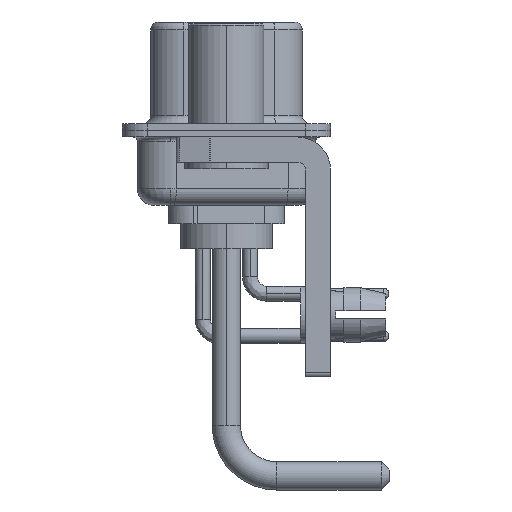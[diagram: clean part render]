
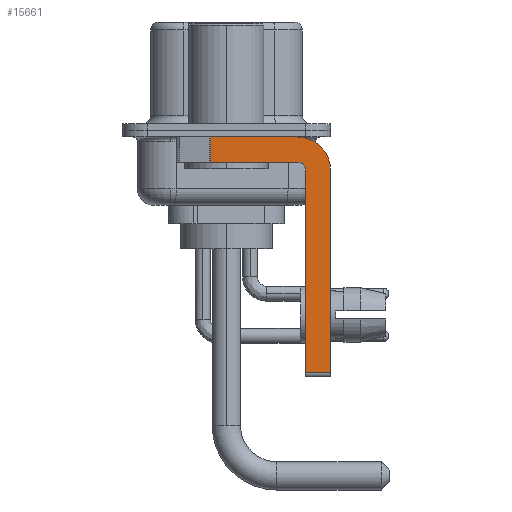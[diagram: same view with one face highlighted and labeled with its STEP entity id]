
A CAD part, left-side view. The second image highlights one B-rep face of the part: STEP entity #15661.
In plain terms, the highlighted planar face has unit normal (-1, 0, 0).
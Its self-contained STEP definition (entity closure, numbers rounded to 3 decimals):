
#631 = LINE ( 'NONE', #7253, #27463 ) ;
#889 = CARTESIAN_POINT ( 'NONE',  ( -2.9, -6.25, -2.4 ) ) ;
#1172 = CARTESIAN_POINT ( 'NONE',  ( -2.9, -4.25, -1.9 ) ) ;
#1406 = CARTESIAN_POINT ( 'NONE',  ( -2.9, 0.978, -0.4 ) ) ;
#1582 = CARTESIAN_POINT ( 'NONE',  ( -2.9, -6.25, -14.55 ) ) ;
#1620 = ORIENTED_EDGE ( 'NONE', *, *, #12519, .T. ) ;
#1623 = LINE ( 'NONE', #1172, #14168 ) ;
#1681 = CARTESIAN_POINT ( 'NONE',  ( -2.9, -4.25, -0.4 ) ) ;
#2259 = CARTESIAN_POINT ( 'NONE',  ( -2.9, -4.75, -14.55 ) ) ;
#2605 = FACE_OUTER_BOUND ( 'NONE', #25635, .T. ) ;
#3520 = AXIS2_PLACEMENT_3D ( 'NONE', #10503, #19725, #3733 ) ;
#3727 = DIRECTION ( 'NONE',  ( 0., 1., 0. ) ) ;
#3733 = DIRECTION ( 'NONE',  ( 0., 0., 1. ) ) ;
#3765 = CARTESIAN_POINT ( 'NONE',  ( -2.9, -4.75, -14.8 ) ) ;
#3868 = VERTEX_POINT ( 'NONE', #1681 ) ;
#4500 = CIRCLE ( 'NONE', #3520, 0.5 ) ;
#4700 = CARTESIAN_POINT ( 'NONE',  ( -2.9, -4.25, -2.4 ) ) ;
#5688 = ORIENTED_EDGE ( 'NONE', *, *, #22179, .F. ) ;
#6718 = VECTOR ( 'NONE', #12790, 1000. ) ;
#7138 = CIRCLE ( 'NONE', #11491, 2. ) ;
#7253 = CARTESIAN_POINT ( 'NONE',  ( -2.9, 0.978, -1.9 ) ) ;
#7730 = EDGE_CURVE ( 'NONE', #3868, #24630, #7138, .T. ) ;
#8283 = LINE ( 'NONE', #17500, #25373 ) ;
#8854 = AXIS2_PLACEMENT_3D ( 'NONE', #9529, #25080, #21013 ) ;
#9052 = VECTOR ( 'NONE', #28943, 1000. ) ;
#9529 = CARTESIAN_POINT ( 'NONE',  ( -2.9, -4.25, -2.4 ) ) ;
#10006 = VERTEX_POINT ( 'NONE', #2259 ) ;
#10503 = CARTESIAN_POINT ( 'NONE',  ( -2.9, -4.25, -2.4 ) ) ;
#11000 = VERTEX_POINT ( 'NONE', #22795 ) ;
#11276 = EDGE_CURVE ( 'NONE', #25109, #3868, #20034, .T. ) ;
#11377 = ORIENTED_EDGE ( 'NONE', *, *, #19997, .F. ) ;
#11491 = AXIS2_PLACEMENT_3D ( 'NONE', #4700, #16015, #27590 ) ;
#12097 = ORIENTED_EDGE ( 'NONE', *, *, #15043, .F. ) ;
#12519 = EDGE_CURVE ( 'NONE', #25109, #15538, #631, .T. ) ;
#12790 = DIRECTION ( 'NONE',  ( 0., -1., 0. ) ) ;
#12973 = DIRECTION ( 'NONE',  ( 0., -1., 0. ) ) ;
#13125 = DIRECTION ( 'NONE',  ( 0., 0., 1. ) ) ;
#13422 = LINE ( 'NONE', #3765, #21462 ) ;
#13546 = ORIENTED_EDGE ( 'NONE', *, *, #7730, .F. ) ;
#14168 = VECTOR ( 'NONE', #3727, 1000. ) ;
#15043 = EDGE_CURVE ( 'NONE', #11000, #16773, #4500, .T. ) ;
#15538 = VERTEX_POINT ( 'NONE', #18172 ) ;
#15661 = ADVANCED_FACE ( 'NONE', ( #2605 ), #20866, .F. ) ;
#16015 = DIRECTION ( 'NONE',  ( 1., 0., 0. ) ) ;
#16773 = VERTEX_POINT ( 'NONE', #18974 ) ;
#17500 = CARTESIAN_POINT ( 'NONE',  ( -2.9, -4.25, -14.55 ) ) ;
#17812 = EDGE_CURVE ( 'NONE', #10006, #18121, #8283, .T. ) ;
#18121 = VERTEX_POINT ( 'NONE', #1582 ) ;
#18172 = CARTESIAN_POINT ( 'NONE',  ( -2.9, 0.978, -1.9 ) ) ;
#18974 = CARTESIAN_POINT ( 'NONE',  ( -2.9, -4.25, -1.9 ) ) ;
#19725 = DIRECTION ( 'NONE',  ( -1., 0., 0. ) ) ;
#19997 = EDGE_CURVE ( 'NONE', #24630, #18121, #22343, .T. ) ;
#20034 = LINE ( 'NONE', #28893, #6718 ) ;
#20866 = PLANE ( 'NONE',  #8854 ) ;
#21013 = DIRECTION ( 'NONE',  ( 0., 0., -1. ) ) ;
#21462 = VECTOR ( 'NONE', #13125, 1000. ) ;
#22179 = EDGE_CURVE ( 'NONE', #10006, #11000, #13422, .T. ) ;
#22343 = LINE ( 'NONE', #29407, #9052 ) ;
#22562 = EDGE_CURVE ( 'NONE', #16773, #15538, #1623, .T. ) ;
#22795 = CARTESIAN_POINT ( 'NONE',  ( -2.9, -4.75, -2.4 ) ) ;
#23707 = ORIENTED_EDGE ( 'NONE', *, *, #22562, .F. ) ;
#24630 = VERTEX_POINT ( 'NONE', #889 ) ;
#25080 = DIRECTION ( 'NONE',  ( 1., 0., 0. ) ) ;
#25109 = VERTEX_POINT ( 'NONE', #1406 ) ;
#25373 = VECTOR ( 'NONE', #12973, 1000. ) ;
#25635 = EDGE_LOOP ( 'NONE', ( #29697, #1620, #23707, #12097, #5688, #27442, #11377, #13546 ) ) ;
#27442 = ORIENTED_EDGE ( 'NONE', *, *, #17812, .T. ) ;
#27463 = VECTOR ( 'NONE', #28338, 1000. ) ;
#27590 = DIRECTION ( 'NONE',  ( 0., 0., -1. ) ) ;
#28338 = DIRECTION ( 'NONE',  ( 0., 0., -1. ) ) ;
#28893 = CARTESIAN_POINT ( 'NONE',  ( -2.9, 3., -0.4 ) ) ;
#28943 = DIRECTION ( 'NONE',  ( 0., 0., -1. ) ) ;
#29407 = CARTESIAN_POINT ( 'NONE',  ( -2.9, -6.25, -2.4 ) ) ;
#29697 = ORIENTED_EDGE ( 'NONE', *, *, #11276, .F. ) ;
